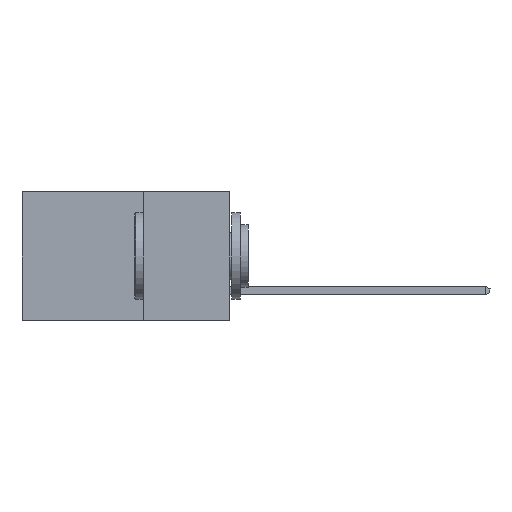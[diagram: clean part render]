
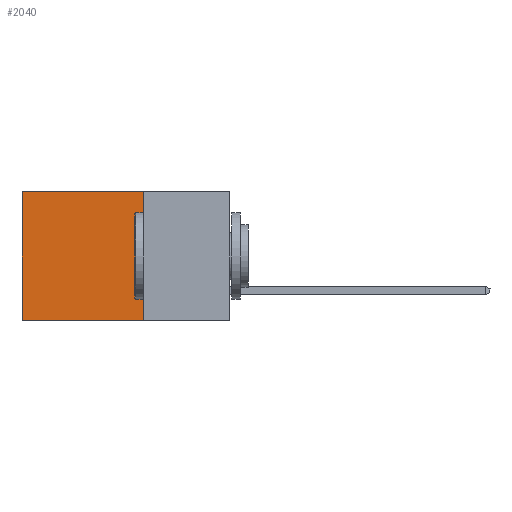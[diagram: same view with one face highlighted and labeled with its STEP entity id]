
A CAD part, left-side view. The second image highlights one B-rep face of the part: STEP entity #2040.
In plain terms, the highlighted planar face has unit normal (-1, 0, 0).
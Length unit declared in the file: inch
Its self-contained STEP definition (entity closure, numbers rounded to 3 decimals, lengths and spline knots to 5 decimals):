
#764 = ORIENTED_EDGE ( 'NONE', *, *, #17944, .T. ) ;
#825 = EDGE_CURVE ( 'NONE', #4074, #19775, #8293, .T. ) ;
#2040 = ADVANCED_FACE ( 'NONE', ( #11760 ), #18287, .F. ) ;
#2374 = DIRECTION ( 'NONE',  ( 0., 0., -1. ) ) ;
#2802 = VECTOR ( 'NONE', #11543, 39.37008 ) ;
#2890 = CARTESIAN_POINT ( 'NONE',  ( 0.2615, 0.25, -0.37 ) ) ;
#3246 = VECTOR ( 'NONE', #9714, 39.37008 ) ;
#3620 = CARTESIAN_POINT ( 'NONE',  ( 0.2615, 0.6, 0. ) ) ;
#4074 = VERTEX_POINT ( 'NONE', #3620 ) ;
#4130 = LINE ( 'NONE', #13172, #2802 ) ;
#4684 = ORIENTED_EDGE ( 'NONE', *, *, #825, .T. ) ;
#5291 = CARTESIAN_POINT ( 'NONE',  ( 0.2615, 0.25, -0.37 ) ) ;
#7209 = EDGE_CURVE ( 'NONE', #17906, #8530, #10099, .T. ) ;
#7459 = LINE ( 'NONE', #2890, #8637 ) ;
#8293 = LINE ( 'NONE', #19164, #3246 ) ;
#8530 = VERTEX_POINT ( 'NONE', #5291 ) ;
#8637 = VECTOR ( 'NONE', #20074, 39.37008 ) ;
#8790 = AXIS2_PLACEMENT_3D ( 'NONE', #15132, #16668, #18088 ) ;
#9714 = DIRECTION ( 'NONE',  ( 0., 0., -1. ) ) ;
#10099 = LINE ( 'NONE', #16304, #11713 ) ;
#11543 = DIRECTION ( 'NONE',  ( 0., 1., 0. ) ) ;
#11713 = VECTOR ( 'NONE', #2374, 39.37008 ) ;
#11760 = FACE_OUTER_BOUND ( 'NONE', #18417, .T. ) ;
#12970 = ORIENTED_EDGE ( 'NONE', *, *, #17294, .F. ) ;
#13172 = CARTESIAN_POINT ( 'NONE',  ( 0.2615, 0.25, 0. ) ) ;
#15132 = CARTESIAN_POINT ( 'NONE',  ( 0.2615, 0.25, -0.37 ) ) ;
#16304 = CARTESIAN_POINT ( 'NONE',  ( 0.2615, 0.25, -0.37 ) ) ;
#16668 = DIRECTION ( 'NONE',  ( 1., 0., 0. ) ) ;
#16715 = ORIENTED_EDGE ( 'NONE', *, *, #7209, .F. ) ;
#17294 = EDGE_CURVE ( 'NONE', #8530, #19775, #7459, .T. ) ;
#17906 = VERTEX_POINT ( 'NONE', #19489 ) ;
#17944 = EDGE_CURVE ( 'NONE', #17906, #4074, #4130, .T. ) ;
#18088 = DIRECTION ( 'NONE',  ( 0., 0., -1. ) ) ;
#18287 = PLANE ( 'NONE',  #8790 ) ;
#18417 = EDGE_LOOP ( 'NONE', ( #4684, #12970, #16715, #764 ) ) ;
#19164 = CARTESIAN_POINT ( 'NONE',  ( 0.2615, 0.6, -0.37 ) ) ;
#19489 = CARTESIAN_POINT ( 'NONE',  ( 0.2615, 0.25, 0. ) ) ;
#19775 = VERTEX_POINT ( 'NONE', #19810 ) ;
#19810 = CARTESIAN_POINT ( 'NONE',  ( 0.2615, 0.6, -0.37 ) ) ;
#20074 = DIRECTION ( 'NONE',  ( 0., 1., 0. ) ) ;
